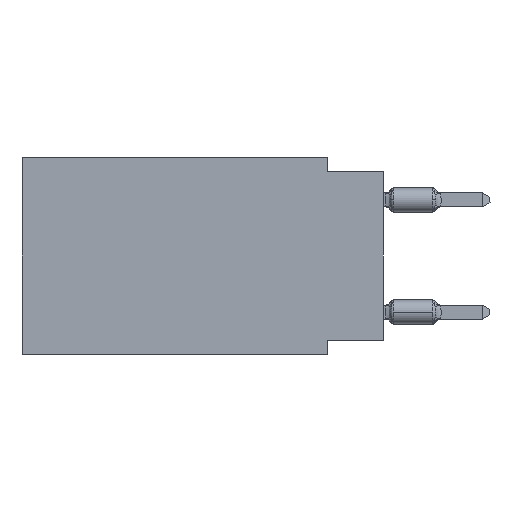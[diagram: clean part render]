
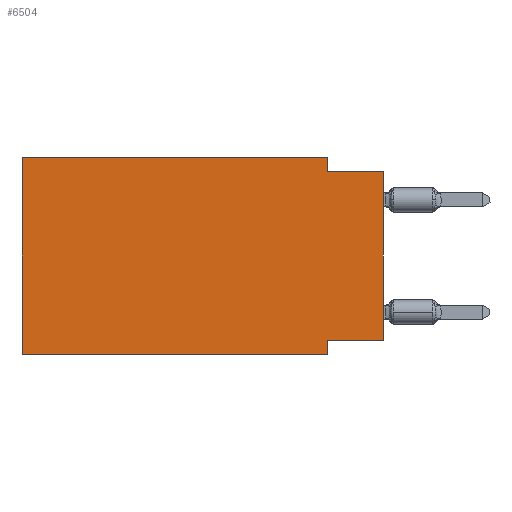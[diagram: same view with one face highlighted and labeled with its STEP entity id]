
A CAD part, left-side view. The second image highlights one B-rep face of the part: STEP entity #6504.
In plain terms, the highlighted planar face has unit normal (-1, 0, 0).
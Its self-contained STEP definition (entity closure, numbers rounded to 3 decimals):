
#659 = VECTOR ( 'NONE', #928, 1000. ) ;
#796 = DIRECTION ( 'NONE',  ( 1., 0., 0. ) ) ;
#928 = DIRECTION ( 'NONE',  ( 0., 1., 0. ) ) ;
#1095 = CARTESIAN_POINT ( 'NONE',  ( 0., 16.383, 0. ) ) ;
#1307 = ORIENTED_EDGE ( 'NONE', *, *, #2425, .F. ) ;
#1435 = CARTESIAN_POINT ( 'NONE',  ( 0., 2.54, 0. ) ) ;
#2348 = DIRECTION ( 'NONE',  ( 0., 0., -1. ) ) ;
#2404 = ORIENTED_EDGE ( 'NONE', *, *, #3939, .F. ) ;
#2418 = VERTEX_POINT ( 'NONE', #7324 ) ;
#2425 = EDGE_CURVE ( 'NONE', #5996, #2418, #4367, .T. ) ;
#2427 = ORIENTED_EDGE ( 'NONE', *, *, #10386, .T. ) ;
#2636 = VECTOR ( 'NONE', #10021, 1000. ) ;
#2735 = CARTESIAN_POINT ( 'NONE',  ( 0., 16.383, -8.89 ) ) ;
#2920 = DIRECTION ( 'NONE',  ( 0., -1., 0. ) ) ;
#3631 = VERTEX_POINT ( 'NONE', #17245 ) ;
#3676 = DIRECTION ( 'NONE',  ( 0., 0., -1. ) ) ;
#3692 = DIRECTION ( 'NONE',  ( 0., -1., 0. ) ) ;
#3739 = LINE ( 'NONE', #15068, #8176 ) ;
#3939 = EDGE_CURVE ( 'NONE', #2418, #17685, #10735, .T. ) ;
#4163 = ORIENTED_EDGE ( 'NONE', *, *, #9891, .F. ) ;
#4367 = LINE ( 'NONE', #15780, #2636 ) ;
#4984 = DIRECTION ( 'NONE',  ( 0., 0., -1. ) ) ;
#5255 = PLANE ( 'NONE',  #14525 ) ;
#5996 = VERTEX_POINT ( 'NONE', #10288 ) ;
#6109 = CARTESIAN_POINT ( 'NONE',  ( 0., 0., 0. ) ) ;
#6192 = EDGE_CURVE ( 'NONE', #3631, #13073, #6572, .T. ) ;
#6366 = CARTESIAN_POINT ( 'NONE',  ( 0., 16.383, 0. ) ) ;
#6504 = ADVANCED_FACE ( 'NONE', ( #9326 ), #5255, .F. ) ;
#6572 = LINE ( 'NONE', #12240, #12081 ) ;
#7324 = CARTESIAN_POINT ( 'NONE',  ( 0., 16.383, 0. ) ) ;
#7493 = ORIENTED_EDGE ( 'NONE', *, *, #17028, .T. ) ;
#7494 = LINE ( 'NONE', #6109, #17751 ) ;
#8056 = DIRECTION ( 'NONE',  ( 0., -1., 0. ) ) ;
#8176 = VECTOR ( 'NONE', #2348, 1000. ) ;
#8204 = VECTOR ( 'NONE', #3676, 1000. ) ;
#8981 = DIRECTION ( 'NONE',  ( 0., 0., 1. ) ) ;
#9326 = FACE_OUTER_BOUND ( 'NONE', #12014, .T. ) ;
#9891 = EDGE_CURVE ( 'NONE', #14560, #10186, #13745, .T. ) ;
#10002 = CARTESIAN_POINT ( 'NONE',  ( 0., 0., -8.255 ) ) ;
#10021 = DIRECTION ( 'NONE',  ( 0., 0., 1. ) ) ;
#10142 = LINE ( 'NONE', #2735, #12539 ) ;
#10186 = VERTEX_POINT ( 'NONE', #10374 ) ;
#10288 = CARTESIAN_POINT ( 'NONE',  ( 0., 16.383, -8.89 ) ) ;
#10374 = CARTESIAN_POINT ( 'NONE',  ( 0., 2.54, -8.255 ) ) ;
#10386 = EDGE_CURVE ( 'NONE', #5996, #11245, #10142, .T. ) ;
#10715 = CARTESIAN_POINT ( 'NONE',  ( 0., 2.54, -8.89 ) ) ;
#10735 = LINE ( 'NONE', #1095, #13846 ) ;
#11245 = VERTEX_POINT ( 'NONE', #13247 ) ;
#12014 = EDGE_LOOP ( 'NONE', ( #7493, #15669, #15985, #2404, #1307, #2427, #16784, #4163 ) ) ;
#12081 = VECTOR ( 'NONE', #8056, 1000. ) ;
#12240 = CARTESIAN_POINT ( 'NONE',  ( 0., 0., -0.635 ) ) ;
#12539 = VECTOR ( 'NONE', #2920, 1000. ) ;
#13073 = VERTEX_POINT ( 'NONE', #16408 ) ;
#13247 = CARTESIAN_POINT ( 'NONE',  ( 0., 2.54, -8.89 ) ) ;
#13745 = LINE ( 'NONE', #17919, #659 ) ;
#13846 = VECTOR ( 'NONE', #3692, 1000. ) ;
#13898 = EDGE_CURVE ( 'NONE', #17685, #3631, #3739, .T. ) ;
#14525 = AXIS2_PLACEMENT_3D ( 'NONE', #6366, #796, #4984 ) ;
#14560 = VERTEX_POINT ( 'NONE', #10002 ) ;
#14683 = EDGE_CURVE ( 'NONE', #10186, #11245, #14995, .T. ) ;
#14995 = LINE ( 'NONE', #10715, #8204 ) ;
#15068 = CARTESIAN_POINT ( 'NONE',  ( 0., 2.54, 0. ) ) ;
#15669 = ORIENTED_EDGE ( 'NONE', *, *, #6192, .F. ) ;
#15780 = CARTESIAN_POINT ( 'NONE',  ( 0., 16.383, 0. ) ) ;
#15985 = ORIENTED_EDGE ( 'NONE', *, *, #13898, .F. ) ;
#16408 = CARTESIAN_POINT ( 'NONE',  ( 0., 0., -0.635 ) ) ;
#16784 = ORIENTED_EDGE ( 'NONE', *, *, #14683, .F. ) ;
#17028 = EDGE_CURVE ( 'NONE', #14560, #13073, #7494, .T. ) ;
#17245 = CARTESIAN_POINT ( 'NONE',  ( 0., 2.54, -0.635 ) ) ;
#17685 = VERTEX_POINT ( 'NONE', #1435 ) ;
#17751 = VECTOR ( 'NONE', #8981, 1000. ) ;
#17919 = CARTESIAN_POINT ( 'NONE',  ( 0., 0., -8.255 ) ) ;
